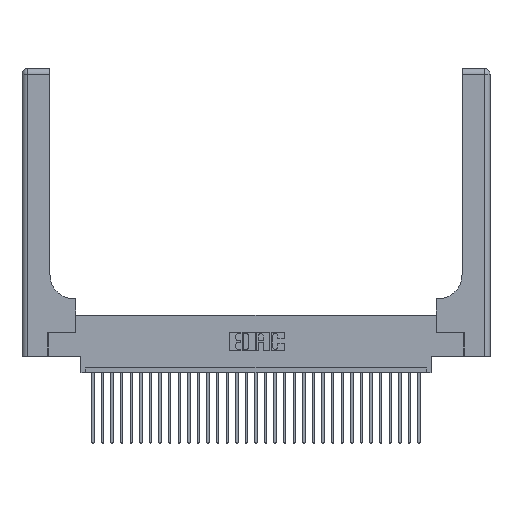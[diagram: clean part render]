
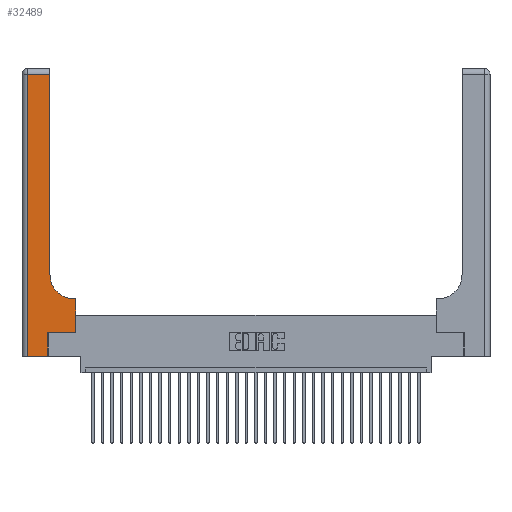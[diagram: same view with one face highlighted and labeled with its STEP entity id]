
A CAD part, top view. The second image highlights one B-rep face of the part: STEP entity #32489.
In plain terms, the highlighted planar face has unit normal (0, 0, 1).
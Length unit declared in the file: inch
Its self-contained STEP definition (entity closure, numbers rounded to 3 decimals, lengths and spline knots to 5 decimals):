
#248 = DIRECTION ( 'NONE',  ( 1., 0., 0. ) ) ;
#444 = LINE ( 'NONE', #9016, #11501 ) ;
#825 = EDGE_CURVE ( 'NONE', #26541, #16489, #30356, .T. ) ;
#1811 = LINE ( 'NONE', #32188, #24285 ) ;
#1897 = VERTEX_POINT ( 'NONE', #32249 ) ;
#2203 = CARTESIAN_POINT ( 'NONE',  ( 0., 0., 0.37 ) ) ;
#2477 = CARTESIAN_POINT ( 'NONE',  ( 0.269, 0.25, 0.37 ) ) ;
#2961 = ORIENTED_EDGE ( 'NONE', *, *, #30204, .T. ) ;
#3341 = ORIENTED_EDGE ( 'NONE', *, *, #11107, .T. ) ;
#3831 = EDGE_CURVE ( 'NONE', #21826, #10733, #7715, .T. ) ;
#4296 = EDGE_CURVE ( 'NONE', #5818, #1897, #19525, .T. ) ;
#4692 = CARTESIAN_POINT ( 'NONE',  ( 0.2915, 2.94, 0.37 ) ) ;
#4755 = DIRECTION ( 'NONE',  ( 1., 0., 0. ) ) ;
#5451 = DIRECTION ( 'NONE',  ( 0., 1., 0. ) ) ;
#5685 = VECTOR ( 'NONE', #4755, 39.37008 ) ;
#5818 = VERTEX_POINT ( 'NONE', #23236 ) ;
#7715 = LINE ( 'NONE', #31222, #19157 ) ;
#8240 = EDGE_LOOP ( 'NONE', ( #22517, #3341, #15198, #30871, #2961, #8703, #10724, #13990, #21800 ) ) ;
#8289 = EDGE_CURVE ( 'NONE', #1897, #21826, #1811, .T. ) ;
#8628 = FACE_OUTER_BOUND ( 'NONE', #8240, .T. ) ;
#8703 = ORIENTED_EDGE ( 'NONE', *, *, #4296, .T. ) ;
#8796 = CARTESIAN_POINT ( 'NONE',  ( 0.06, 2.94, 0.37 ) ) ;
#9016 = CARTESIAN_POINT ( 'NONE',  ( 0.269, 0., 0.37 ) ) ;
#9738 = LINE ( 'NONE', #18518, #20364 ) ;
#10086 = DIRECTION ( 'NONE',  ( 0., -1., 0. ) ) ;
#10159 = PLANE ( 'NONE',  #31501 ) ;
#10172 = DIRECTION ( 'NONE',  ( 0., 0., -1. ) ) ;
#10277 = CARTESIAN_POINT ( 'NONE',  ( 0.2915, 3., 0.37 ) ) ;
#10419 = CARTESIAN_POINT ( 'NONE',  ( 0.06, 0., 0.37 ) ) ;
#10724 = ORIENTED_EDGE ( 'NONE', *, *, #8289, .T. ) ;
#10733 = VERTEX_POINT ( 'NONE', #14878 ) ;
#11107 = EDGE_CURVE ( 'NONE', #19746, #26541, #9738, .T. ) ;
#11501 = VECTOR ( 'NONE', #16474, 39.37008 ) ;
#12822 = VECTOR ( 'NONE', #29957, 39.37008 ) ;
#12938 = VERTEX_POINT ( 'NONE', #27621 ) ;
#13028 = VECTOR ( 'NONE', #10086, 39.37008 ) ;
#13222 = DIRECTION ( 'NONE',  ( -1., 0., 0. ) ) ;
#13990 = ORIENTED_EDGE ( 'NONE', *, *, #3831, .T. ) ;
#14878 = CARTESIAN_POINT ( 'NONE',  ( 0.5415, 0.6, 0.37 ) ) ;
#15198 = ORIENTED_EDGE ( 'NONE', *, *, #825, .T. ) ;
#15546 = CARTESIAN_POINT ( 'NONE',  ( 0., 3., 0.37 ) ) ;
#15604 = VERTEX_POINT ( 'NONE', #30832 ) ;
#16474 = DIRECTION ( 'NONE',  ( 0., 1., 0. ) ) ;
#16489 = VERTEX_POINT ( 'NONE', #10419 ) ;
#16753 = AXIS2_PLACEMENT_3D ( 'NONE', #20298, #10172, #248 ) ;
#18248 = LINE ( 'NONE', #2203, #5685 ) ;
#18518 = CARTESIAN_POINT ( 'NONE',  ( 0., 2.94, 0.37 ) ) ;
#18666 = DIRECTION ( 'NONE',  ( -1., 0., 0. ) ) ;
#18832 = DIRECTION ( 'NONE',  ( 0., 1., 0. ) ) ;
#19157 = VECTOR ( 'NONE', #18666, 39.37008 ) ;
#19525 = LINE ( 'NONE', #2477, #12822 ) ;
#19746 = VERTEX_POINT ( 'NONE', #4692 ) ;
#20285 = DIRECTION ( 'NONE',  ( -1., 0., 0. ) ) ;
#20298 = CARTESIAN_POINT ( 'NONE',  ( 0.5415, 0.85, 0.37 ) ) ;
#20364 = VECTOR ( 'NONE', #13222, 39.37008 ) ;
#21800 = ORIENTED_EDGE ( 'NONE', *, *, #21928, .T. ) ;
#21826 = VERTEX_POINT ( 'NONE', #27639 ) ;
#21894 = EDGE_CURVE ( 'NONE', #12938, #19746, #24385, .T. ) ;
#21928 = EDGE_CURVE ( 'NONE', #10733, #12938, #23570, .T. ) ;
#22517 = ORIENTED_EDGE ( 'NONE', *, *, #21894, .T. ) ;
#22794 = VECTOR ( 'NONE', #5451, 39.37008 ) ;
#22963 = CARTESIAN_POINT ( 'NONE',  ( 0.06, 3., 0.37 ) ) ;
#23236 = CARTESIAN_POINT ( 'NONE',  ( 0.269, 0.25, 0.37 ) ) ;
#23570 = CIRCLE ( 'NONE', #16753, 0.25 ) ;
#24285 = VECTOR ( 'NONE', #18832, 39.37008 ) ;
#24385 = LINE ( 'NONE', #10277, #22794 ) ;
#26541 = VERTEX_POINT ( 'NONE', #8796 ) ;
#27621 = CARTESIAN_POINT ( 'NONE',  ( 0.2915, 0.85, 0.37 ) ) ;
#27639 = CARTESIAN_POINT ( 'NONE',  ( 0.5585, 0.6, 0.37 ) ) ;
#28338 = EDGE_CURVE ( 'NONE', #16489, #15604, #18248, .T. ) ;
#29957 = DIRECTION ( 'NONE',  ( 1., 0., 0. ) ) ;
#30204 = EDGE_CURVE ( 'NONE', #15604, #5818, #444, .T. ) ;
#30356 = LINE ( 'NONE', #22963, #13028 ) ;
#30385 = DIRECTION ( 'NONE',  ( 0., 0., -1. ) ) ;
#30832 = CARTESIAN_POINT ( 'NONE',  ( 0.269, 0., 0.37 ) ) ;
#30871 = ORIENTED_EDGE ( 'NONE', *, *, #28338, .T. ) ;
#31222 = CARTESIAN_POINT ( 'NONE',  ( 0.2915, 0.6, 0.37 ) ) ;
#31501 = AXIS2_PLACEMENT_3D ( 'NONE', #15546, #30385, #20285 ) ;
#32188 = CARTESIAN_POINT ( 'NONE',  ( 0.5585, 0.25, 0.37 ) ) ;
#32249 = CARTESIAN_POINT ( 'NONE',  ( 0.5585, 0.25, 0.37 ) ) ;
#32489 = ADVANCED_FACE ( 'NONE', ( #8628 ), #10159, .F. ) ;
